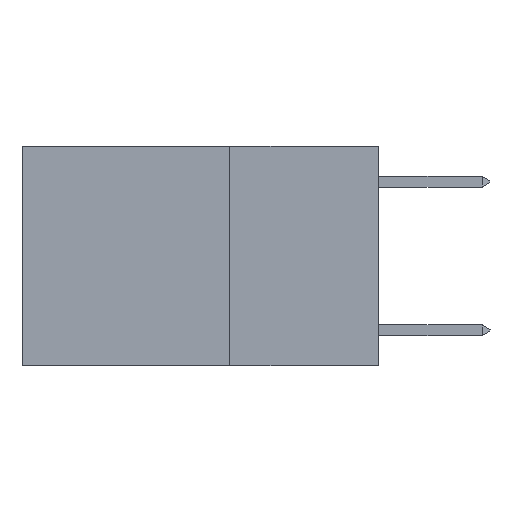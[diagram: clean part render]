
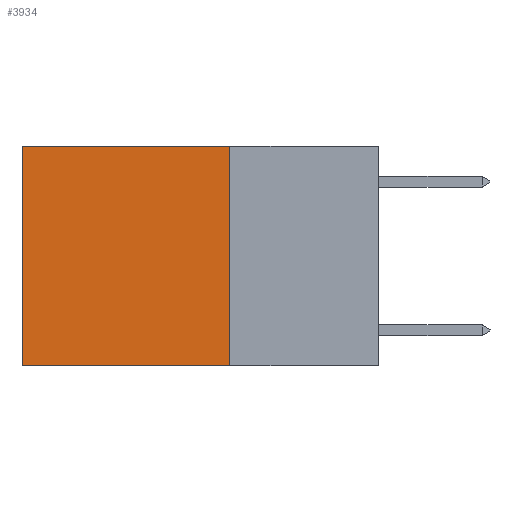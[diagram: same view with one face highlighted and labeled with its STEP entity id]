
A CAD part, left-side view. The second image highlights one B-rep face of the part: STEP entity #3934.
In plain terms, the highlighted planar face has unit normal (-1, 0, 0).
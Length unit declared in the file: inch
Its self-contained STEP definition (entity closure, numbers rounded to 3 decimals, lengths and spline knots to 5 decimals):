
#27 = DIRECTION ( 'NONE',  ( 0., 1., 0. ) ) ;
#446 = EDGE_CURVE ( 'NONE', #2373, #3300, #2270, .T. ) ;
#620 = EDGE_CURVE ( 'NONE', #6597, #10126, #7771, .T. ) ;
#987 = VECTOR ( 'NONE', #6525, 39.37008 ) ;
#1345 = ORIENTED_EDGE ( 'NONE', *, *, #4051, .F. ) ;
#1738 = EDGE_LOOP ( 'NONE', ( #1779, #1345, #9070, #8049 ) ) ;
#1779 = ORIENTED_EDGE ( 'NONE', *, *, #446, .T. ) ;
#1921 = DIRECTION ( 'NONE',  ( 1., 0., 0. ) ) ;
#2270 = LINE ( 'NONE', #8904, #987 ) ;
#2373 = VERTEX_POINT ( 'NONE', #3494 ) ;
#2601 = CARTESIAN_POINT ( 'NONE',  ( 0.2625, 0.25, -0.37 ) ) ;
#2618 = CARTESIAN_POINT ( 'NONE',  ( 0.2625, 0.25, 0. ) ) ;
#3300 = VERTEX_POINT ( 'NONE', #5827 ) ;
#3456 = EDGE_CURVE ( 'NONE', #6597, #2373, #4380, .T. ) ;
#3494 = CARTESIAN_POINT ( 'NONE',  ( 0.2625, 0.6, 0. ) ) ;
#3541 = CARTESIAN_POINT ( 'NONE',  ( 0.2625, 0.25, 0. ) ) ;
#3737 = FACE_OUTER_BOUND ( 'NONE', #1738, .T. ) ;
#3934 = ADVANCED_FACE ( 'NONE', ( #3737 ), #8263, .F. ) ;
#4013 = VECTOR ( 'NONE', #27, 39.37008 ) ;
#4051 = EDGE_CURVE ( 'NONE', #10126, #3300, #6687, .T. ) ;
#4380 = LINE ( 'NONE', #2618, #4013 ) ;
#4955 = VECTOR ( 'NONE', #10145, 39.37008 ) ;
#5087 = AXIS2_PLACEMENT_3D ( 'NONE', #6810, #1921, #6032 ) ;
#5827 = CARTESIAN_POINT ( 'NONE',  ( 0.2625, 0.6, -0.37 ) ) ;
#6032 = DIRECTION ( 'NONE',  ( 0., 0., -1. ) ) ;
#6525 = DIRECTION ( 'NONE',  ( 0., 0., -1. ) ) ;
#6597 = VERTEX_POINT ( 'NONE', #8629 ) ;
#6687 = LINE ( 'NONE', #2601, #7181 ) ;
#6810 = CARTESIAN_POINT ( 'NONE',  ( 0.2625, 0.25, 0. ) ) ;
#7181 = VECTOR ( 'NONE', #8324, 39.37008 ) ;
#7771 = LINE ( 'NONE', #3541, #4955 ) ;
#7986 = CARTESIAN_POINT ( 'NONE',  ( 0.2625, 0.25, -0.37 ) ) ;
#8049 = ORIENTED_EDGE ( 'NONE', *, *, #3456, .T. ) ;
#8263 = PLANE ( 'NONE',  #5087 ) ;
#8324 = DIRECTION ( 'NONE',  ( 0., 1., 0. ) ) ;
#8629 = CARTESIAN_POINT ( 'NONE',  ( 0.2625, 0.25, 0. ) ) ;
#8904 = CARTESIAN_POINT ( 'NONE',  ( 0.2625, 0.6, 0. ) ) ;
#9070 = ORIENTED_EDGE ( 'NONE', *, *, #620, .F. ) ;
#10126 = VERTEX_POINT ( 'NONE', #7986 ) ;
#10145 = DIRECTION ( 'NONE',  ( 0., 0., -1. ) ) ;
